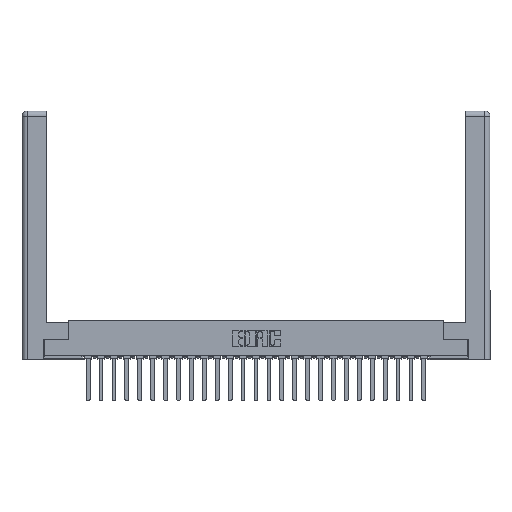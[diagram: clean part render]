
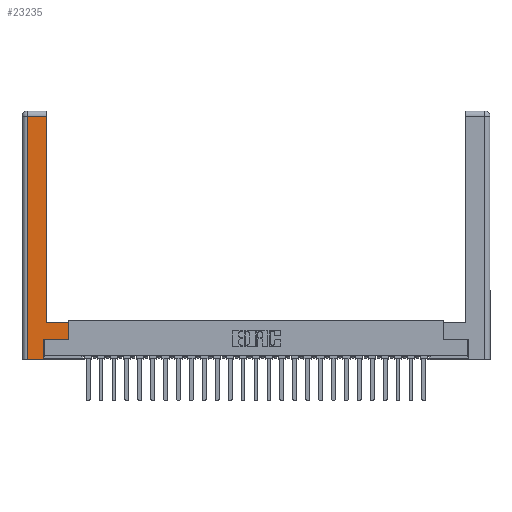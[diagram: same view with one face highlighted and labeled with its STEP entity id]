
A CAD part, top view. The second image highlights one B-rep face of the part: STEP entity #23235.
In plain terms, the highlighted planar face has unit normal (0, 0, 1).
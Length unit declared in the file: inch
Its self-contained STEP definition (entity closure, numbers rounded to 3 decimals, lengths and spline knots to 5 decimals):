
#707 = CARTESIAN_POINT ( 'NONE',  ( 0.295, 3., 0. ) ) ;
#746 = ORIENTED_EDGE ( 'NONE', *, *, #9709, .T. ) ;
#1442 = CARTESIAN_POINT ( 'NONE',  ( 0.265, 0., 0. ) ) ;
#2139 = PLANE ( 'NONE',  #17198 ) ;
#2198 = CARTESIAN_POINT ( 'NONE',  ( 0.565, 0.245, 0. ) ) ;
#2319 = EDGE_CURVE ( 'NONE', #26099, #27716, #4239, .T. ) ;
#2597 = LINE ( 'NONE', #9641, #4646 ) ;
#2900 = DIRECTION ( 'NONE',  ( 0., 0., -1. ) ) ;
#3529 = CARTESIAN_POINT ( 'NONE',  ( 0.0615, 0., 0. ) ) ;
#4213 = LINE ( 'NONE', #707, #20014 ) ;
#4239 = LINE ( 'NONE', #25563, #24769 ) ;
#4600 = ORIENTED_EDGE ( 'NONE', *, *, #21430, .T. ) ;
#4646 = VECTOR ( 'NONE', #7460, 39.37008 ) ;
#5061 = CARTESIAN_POINT ( 'NONE',  ( 0.265, 0.245, 0. ) ) ;
#5794 = LINE ( 'NONE', #3529, #8217 ) ;
#6358 = CARTESIAN_POINT ( 'NONE',  ( 0.0615, 0., 0. ) ) ;
#6986 = ORIENTED_EDGE ( 'NONE', *, *, #10999, .T. ) ;
#7460 = DIRECTION ( 'NONE',  ( -1., 0., 0. ) ) ;
#7468 = DIRECTION ( 'NONE',  ( 0., 1., 0. ) ) ;
#7547 = CARTESIAN_POINT ( 'NONE',  ( 0.295, 0.45, 0. ) ) ;
#7695 = CARTESIAN_POINT ( 'NONE',  ( 0.565, 0.45, 0. ) ) ;
#8100 = VERTEX_POINT ( 'NONE', #13094 ) ;
#8217 = VECTOR ( 'NONE', #10277, 39.37008 ) ;
#8599 = EDGE_CURVE ( 'NONE', #16537, #8100, #21595, .T. ) ;
#8660 = VECTOR ( 'NONE', #24085, 39.37008 ) ;
#9006 = ORIENTED_EDGE ( 'NONE', *, *, #2319, .T. ) ;
#9641 = CARTESIAN_POINT ( 'NONE',  ( 0.295, 0.45, 0. ) ) ;
#9709 = EDGE_CURVE ( 'NONE', #27716, #9816, #2597, .T. ) ;
#9816 = VERTEX_POINT ( 'NONE', #7547 ) ;
#10277 = DIRECTION ( 'NONE',  ( 0., -1., 0. ) ) ;
#10999 = EDGE_CURVE ( 'NONE', #9816, #22054, #4213, .T. ) ;
#11346 = EDGE_CURVE ( 'NONE', #22054, #17038, #14118, .T. ) ;
#11430 = ORIENTED_EDGE ( 'NONE', *, *, #11346, .T. ) ;
#12431 = EDGE_CURVE ( 'NONE', #12504, #26099, #21814, .T. ) ;
#12504 = VERTEX_POINT ( 'NONE', #5061 ) ;
#12507 = ORIENTED_EDGE ( 'NONE', *, *, #8599, .T. ) ;
#13090 = CARTESIAN_POINT ( 'NONE',  ( 0.0615, 2.94, 0. ) ) ;
#13094 = CARTESIAN_POINT ( 'NONE',  ( 0.265, 0., 0. ) ) ;
#13368 = CARTESIAN_POINT ( 'NONE',  ( 0., 0., 0. ) ) ;
#13394 = CARTESIAN_POINT ( 'NONE',  ( 0.265, 0.245, 0. ) ) ;
#13442 = LINE ( 'NONE', #13394, #22017 ) ;
#14118 = LINE ( 'NONE', #13090, #8660 ) ;
#15959 = VECTOR ( 'NONE', #17265, 39.37008 ) ;
#16537 = VERTEX_POINT ( 'NONE', #6358 ) ;
#17038 = VERTEX_POINT ( 'NONE', #20530 ) ;
#17198 = AXIS2_PLACEMENT_3D ( 'NONE', #13368, #2900, #22544 ) ;
#17265 = DIRECTION ( 'NONE',  ( 1., 0., 0. ) ) ;
#18850 = CARTESIAN_POINT ( 'NONE',  ( 0.295, 2.94, 0. ) ) ;
#19973 = EDGE_CURVE ( 'NONE', #8100, #12504, #13442, .T. ) ;
#20014 = VECTOR ( 'NONE', #7468, 39.37008 ) ;
#20121 = DIRECTION ( 'NONE',  ( 0., 1., 0. ) ) ;
#20530 = CARTESIAN_POINT ( 'NONE',  ( 0.0615, 2.94, 0. ) ) ;
#21155 = ORIENTED_EDGE ( 'NONE', *, *, #12431, .T. ) ;
#21430 = EDGE_CURVE ( 'NONE', #17038, #16537, #5794, .T. ) ;
#21595 = LINE ( 'NONE', #1442, #23311 ) ;
#21814 = LINE ( 'NONE', #23871, #15959 ) ;
#22017 = VECTOR ( 'NONE', #20121, 39.37008 ) ;
#22054 = VERTEX_POINT ( 'NONE', #18850 ) ;
#22544 = DIRECTION ( 'NONE',  ( -1., 0., 0. ) ) ;
#23235 = ADVANCED_FACE ( 'NONE', ( #26596 ), #2139, .F. ) ;
#23311 = VECTOR ( 'NONE', #25743, 39.37008 ) ;
#23670 = DIRECTION ( 'NONE',  ( 0., 1., 0. ) ) ;
#23871 = CARTESIAN_POINT ( 'NONE',  ( 0.565, 0.245, 0. ) ) ;
#24085 = DIRECTION ( 'NONE',  ( -1., 0., 0. ) ) ;
#24769 = VECTOR ( 'NONE', #23670, 39.37008 ) ;
#25563 = CARTESIAN_POINT ( 'NONE',  ( 0.565, 0.45, 0. ) ) ;
#25743 = DIRECTION ( 'NONE',  ( 1., 0., 0. ) ) ;
#25826 = ORIENTED_EDGE ( 'NONE', *, *, #19973, .T. ) ;
#26099 = VERTEX_POINT ( 'NONE', #2198 ) ;
#26596 = FACE_OUTER_BOUND ( 'NONE', #27503, .T. ) ;
#27503 = EDGE_LOOP ( 'NONE', ( #6986, #11430, #4600, #12507, #25826, #21155, #9006, #746 ) ) ;
#27716 = VERTEX_POINT ( 'NONE', #7695 ) ;
